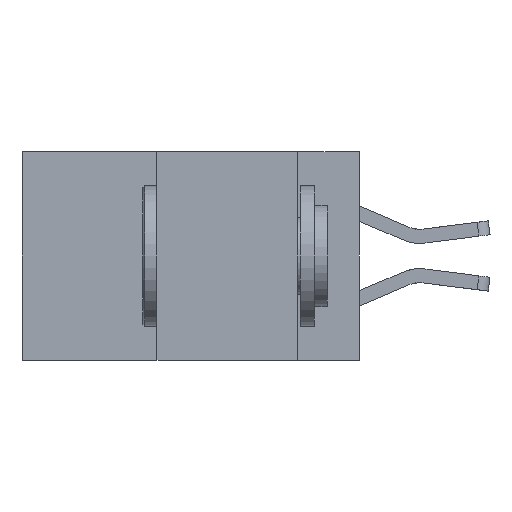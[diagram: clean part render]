
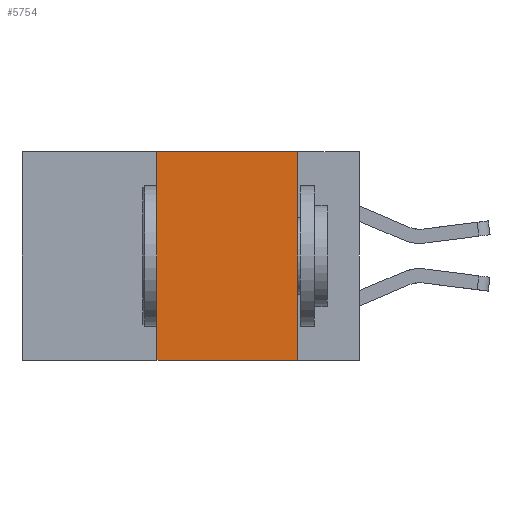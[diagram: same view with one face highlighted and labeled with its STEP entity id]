
A CAD part, left-side view. The second image highlights one B-rep face of the part: STEP entity #5754.
In plain terms, the highlighted planar face has unit normal (-1, 0, 0).
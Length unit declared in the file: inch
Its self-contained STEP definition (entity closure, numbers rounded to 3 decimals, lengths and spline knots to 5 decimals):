
#345 = EDGE_CURVE ( 'NONE', #2306, #14643, #8695, .T. ) ;
#1811 = CARTESIAN_POINT ( 'NONE',  ( 0., 0.36, -0.37 ) ) ;
#2306 = VERTEX_POINT ( 'NONE', #4147 ) ;
#2692 = LINE ( 'NONE', #8686, #15231 ) ;
#3311 = CARTESIAN_POINT ( 'NONE',  ( 0., 0.11, -0.37 ) ) ;
#3912 = DIRECTION ( 'NONE',  ( 0., 0., 1. ) ) ;
#4147 = CARTESIAN_POINT ( 'NONE',  ( 0., 0.11, 0. ) ) ;
#4587 = LINE ( 'NONE', #8291, #8162 ) ;
#4792 = FACE_OUTER_BOUND ( 'NONE', #7970, .T. ) ;
#5754 = ADVANCED_FACE ( 'NONE', ( #4792 ), #8830, .F. ) ;
#5793 = ORIENTED_EDGE ( 'NONE', *, *, #15670, .F. ) ;
#5798 = CARTESIAN_POINT ( 'NONE',  ( 0., 0.6, 0. ) ) ;
#6222 = AXIS2_PLACEMENT_3D ( 'NONE', #8886, #9012, #8803 ) ;
#6995 = DIRECTION ( 'NONE',  ( 0., -1., 0. ) ) ;
#7293 = EDGE_CURVE ( 'NONE', #9316, #14630, #2692, .T. ) ;
#7653 = ORIENTED_EDGE ( 'NONE', *, *, #7293, .F. ) ;
#7970 = EDGE_LOOP ( 'NONE', ( #10253, #5793, #7653, #15674 ) ) ;
#8162 = VECTOR ( 'NONE', #15660, 39.37008 ) ;
#8291 = CARTESIAN_POINT ( 'NONE',  ( 0., 0.6, -0.37 ) ) ;
#8686 = CARTESIAN_POINT ( 'NONE',  ( 0., 0.36, 0. ) ) ;
#8695 = LINE ( 'NONE', #9643, #11154 ) ;
#8803 = DIRECTION ( 'NONE',  ( 0., 0., -1. ) ) ;
#8830 = PLANE ( 'NONE',  #6222 ) ;
#8886 = CARTESIAN_POINT ( 'NONE',  ( 0., 0.6, 0. ) ) ;
#9012 = DIRECTION ( 'NONE',  ( 1., 0., 0. ) ) ;
#9316 = VERTEX_POINT ( 'NONE', #1811 ) ;
#9643 = CARTESIAN_POINT ( 'NONE',  ( 0., 0.11, 0. ) ) ;
#10253 = ORIENTED_EDGE ( 'NONE', *, *, #345, .F. ) ;
#10487 = CARTESIAN_POINT ( 'NONE',  ( 0., 0.36, 0. ) ) ;
#11028 = DIRECTION ( 'NONE',  ( 0., 0., -1. ) ) ;
#11154 = VECTOR ( 'NONE', #11028, 39.37008 ) ;
#12894 = VECTOR ( 'NONE', #6995, 39.37008 ) ;
#14630 = VERTEX_POINT ( 'NONE', #10487 ) ;
#14643 = VERTEX_POINT ( 'NONE', #3311 ) ;
#15231 = VECTOR ( 'NONE', #3912, 39.37008 ) ;
#15660 = DIRECTION ( 'NONE',  ( 0., -1., 0. ) ) ;
#15670 = EDGE_CURVE ( 'NONE', #14630, #2306, #15789, .T. ) ;
#15674 = ORIENTED_EDGE ( 'NONE', *, *, #15748, .T. ) ;
#15748 = EDGE_CURVE ( 'NONE', #9316, #14643, #4587, .T. ) ;
#15789 = LINE ( 'NONE', #5798, #12894 ) ;
